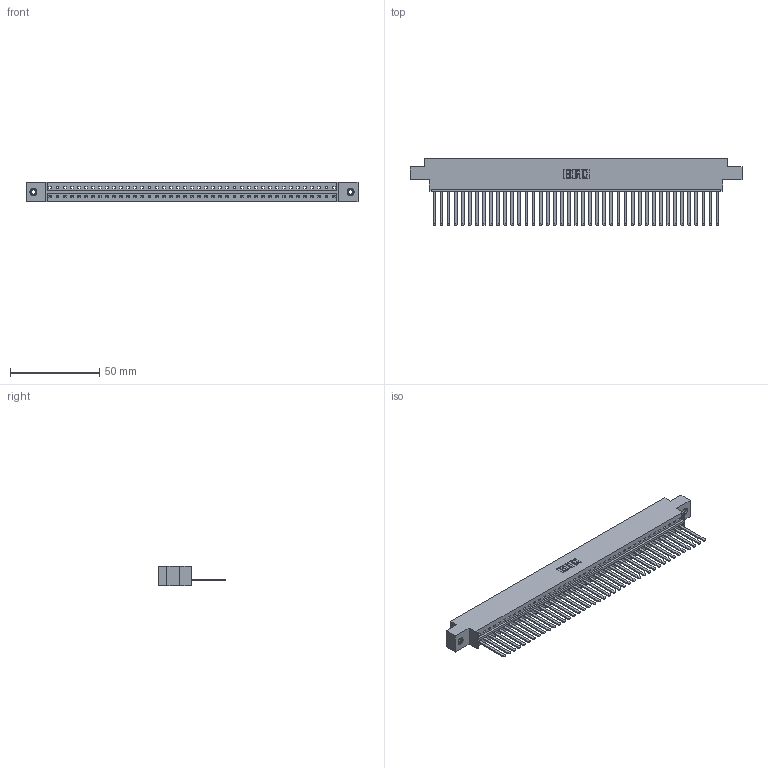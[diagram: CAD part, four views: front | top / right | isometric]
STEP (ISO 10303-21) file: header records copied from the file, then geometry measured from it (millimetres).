
FILE_DESCRIPTION (( 'STEP AP203' ), '1' );
FILE_NAME ('336-041-541-607.STEP', '2020-08-07T23:28:56', ( '' ), ( '' ), 'SwSTEP 2.0', 'SolidWorks 2020', '' );
FILE_SCHEMA (( 'CONFIG_CONTROL_DESIGN' ));
Length unit declared in the file: inch
Products named in the file (4): 336 Part_Offset - .156 Dia - TI; 336-290-001_336-290-541; 345-250-001_345-250-005-103; 336-041-541-607
Assembly tree (44 placements, depth 2):
  336-041-541-607
    336 Part_Offset - .156 Dia - TI
    336-290-001_336-290-541  x41
    345-250-001_345-250-005-103  x2
Bounding box: 185.85 x 37.34 x 11.1 mm (x, y, z)
Volume: 27036 mm3; surface area: 29536.8 mm2
Topology: 44 solids, 44 shells, 2228 faces, 6773 edges, 4480 vertices
Faces by surface type: plane 1500, cylinder 712, cone 12, torus 4
Entity records: 31643 total; most frequent: CARTESIAN_POINT 5575, ORIENTED_EDGE 5446, DIRECTION 4631, EDGE_CURVE 2723, LINE 2571, VECTOR 2571, VERTEX_POINT 1810, AXIS2_PLACEMENT_3D 1030
